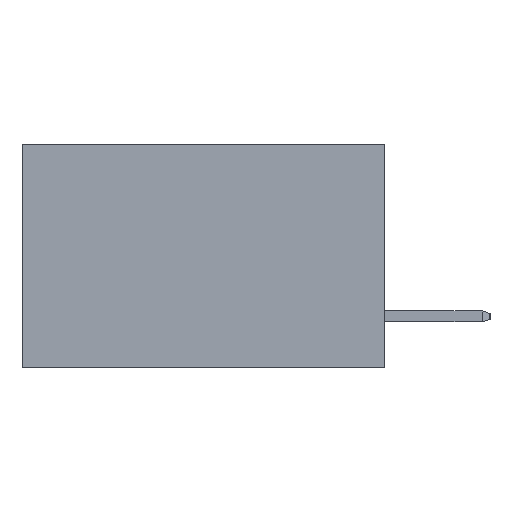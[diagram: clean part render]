
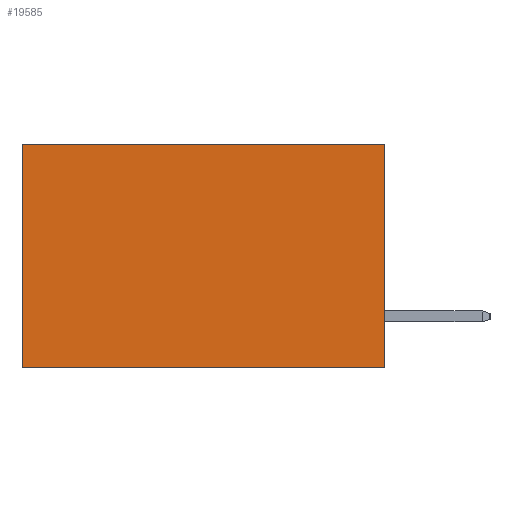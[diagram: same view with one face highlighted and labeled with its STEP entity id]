
A CAD part, left-side view. The second image highlights one B-rep face of the part: STEP entity #19585.
In plain terms, the highlighted planar face has unit normal (-1, 0, 0).
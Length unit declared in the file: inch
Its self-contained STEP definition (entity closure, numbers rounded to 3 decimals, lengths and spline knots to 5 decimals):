
#423 = ORIENTED_EDGE ( 'NONE', *, *, #13961, .T. ) ;
#1443 = ORIENTED_EDGE ( 'NONE', *, *, #6431, .T. ) ;
#2868 = LINE ( 'NONE', #7163, #17245 ) ;
#4232 = LINE ( 'NONE', #11355, #18493 ) ;
#4323 = ORIENTED_EDGE ( 'NONE', *, *, #18564, .F. ) ;
#5367 = EDGE_CURVE ( 'NONE', #14604, #23084, #4232, .T. ) ;
#6261 = DIRECTION ( 'NONE',  ( 0., 0., -1. ) ) ;
#6431 = EDGE_CURVE ( 'NONE', #23299, #8411, #20554, .T. ) ;
#6642 = CARTESIAN_POINT ( 'NONE',  ( 0.2615, 0., 0. ) ) ;
#7163 = CARTESIAN_POINT ( 'NONE',  ( 0.2615, 0., -0.37 ) ) ;
#7877 = CARTESIAN_POINT ( 'NONE',  ( 0.2615, 0., -0.37 ) ) ;
#8411 = VERTEX_POINT ( 'NONE', #17786 ) ;
#8581 = CARTESIAN_POINT ( 'NONE',  ( 0.2615, 0.6, -0.37 ) ) ;
#9101 = ORIENTED_EDGE ( 'NONE', *, *, #5367, .F. ) ;
#10348 = VECTOR ( 'NONE', #6261, 39.37008 ) ;
#10500 = PLANE ( 'NONE',  #14865 ) ;
#10898 = DIRECTION ( 'NONE',  ( 0., 0., -1. ) ) ;
#11355 = CARTESIAN_POINT ( 'NONE',  ( 0.2615, 0., -0.37 ) ) ;
#12251 = CARTESIAN_POINT ( 'NONE',  ( 0.2615, 0., -0.37 ) ) ;
#12330 = DIRECTION ( 'NONE',  ( 0., 0., -1. ) ) ;
#13249 = FACE_OUTER_BOUND ( 'NONE', #13762, .T. ) ;
#13762 = EDGE_LOOP ( 'NONE', ( #1443, #4323, #9101, #423 ) ) ;
#13961 = EDGE_CURVE ( 'NONE', #14604, #23299, #18943, .T. ) ;
#14160 = VECTOR ( 'NONE', #21368, 39.37008 ) ;
#14604 = VERTEX_POINT ( 'NONE', #6642 ) ;
#14865 = AXIS2_PLACEMENT_3D ( 'NONE', #12251, #23118, #12330 ) ;
#17245 = VECTOR ( 'NONE', #21834, 39.37008 ) ;
#17786 = CARTESIAN_POINT ( 'NONE',  ( 0.2615, 0.6, -0.37 ) ) ;
#18493 = VECTOR ( 'NONE', #10898, 39.37008 ) ;
#18564 = EDGE_CURVE ( 'NONE', #23084, #8411, #2868, .T. ) ;
#18943 = LINE ( 'NONE', #19573, #14160 ) ;
#19573 = CARTESIAN_POINT ( 'NONE',  ( 0.2615, 0., 0. ) ) ;
#19585 = ADVANCED_FACE ( 'NONE', ( #13249 ), #10500, .F. ) ;
#20554 = LINE ( 'NONE', #8581, #10348 ) ;
#21318 = CARTESIAN_POINT ( 'NONE',  ( 0.2615, 0.6, 0. ) ) ;
#21368 = DIRECTION ( 'NONE',  ( 0., 1., 0. ) ) ;
#21834 = DIRECTION ( 'NONE',  ( 0., 1., 0. ) ) ;
#23084 = VERTEX_POINT ( 'NONE', #7877 ) ;
#23118 = DIRECTION ( 'NONE',  ( 1., 0., 0. ) ) ;
#23299 = VERTEX_POINT ( 'NONE', #21318 ) ;
